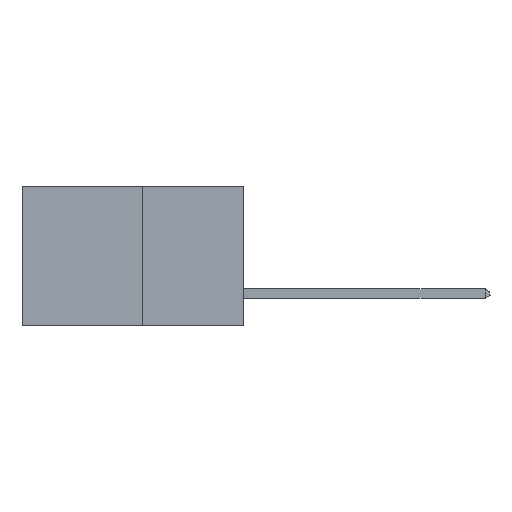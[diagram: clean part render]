
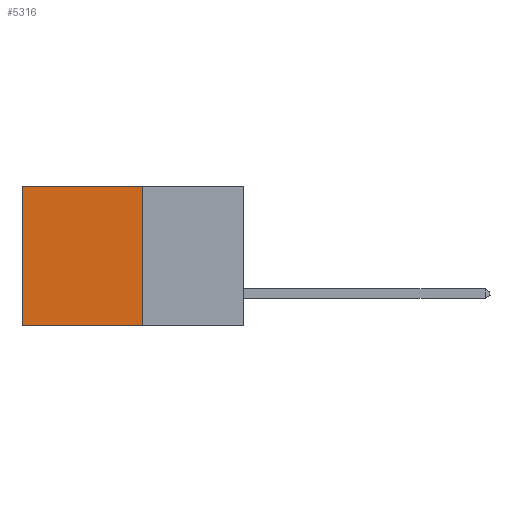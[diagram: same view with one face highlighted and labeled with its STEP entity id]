
A CAD part, left-side view. The second image highlights one B-rep face of the part: STEP entity #5316.
In plain terms, the highlighted planar face has unit normal (-1, 0, 0).
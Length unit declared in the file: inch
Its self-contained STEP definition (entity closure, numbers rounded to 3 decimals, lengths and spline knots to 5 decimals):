
#2037 = DIRECTION ( 'NONE',  ( 0., 0., -1. ) ) ;
#2765 = LINE ( 'NONE', #18623, #16730 ) ;
#3274 = ORIENTED_EDGE ( 'NONE', *, *, #3331, .T. ) ;
#3331 = EDGE_CURVE ( 'NONE', #10796, #9456, #19341, .T. ) ;
#3880 = EDGE_CURVE ( 'NONE', #13641, #21394, #17955, .T. ) ;
#4308 = FACE_OUTER_BOUND ( 'NONE', #7046, .T. ) ;
#5316 = ADVANCED_FACE ( 'NONE', ( #4308 ), #15536, .F. ) ;
#5836 = CARTESIAN_POINT ( 'NONE',  ( 0.277, 0.59, -0.37 ) ) ;
#7046 = EDGE_LOOP ( 'NONE', ( #3274, #19490, #17551, #21540 ) ) ;
#7823 = DIRECTION ( 'NONE',  ( 0., 1., 0. ) ) ;
#9456 = VERTEX_POINT ( 'NONE', #14507 ) ;
#9667 = VECTOR ( 'NONE', #21950, 39.37008 ) ;
#10212 = CARTESIAN_POINT ( 'NONE',  ( 0.277, 0.27, 0. ) ) ;
#10796 = VERTEX_POINT ( 'NONE', #14451 ) ;
#11506 = DIRECTION ( 'NONE',  ( 0., 0., -1. ) ) ;
#11663 = DIRECTION ( 'NONE',  ( 1., 0., 0. ) ) ;
#12351 = CARTESIAN_POINT ( 'NONE',  ( 0.277, 0.27, -0.37 ) ) ;
#13641 = VERTEX_POINT ( 'NONE', #10212 ) ;
#14451 = CARTESIAN_POINT ( 'NONE',  ( 0.277, 0.59, 0. ) ) ;
#14507 = CARTESIAN_POINT ( 'NONE',  ( 0.277, 0.59, -0.37 ) ) ;
#15536 = PLANE ( 'NONE',  #17037 ) ;
#15633 = DIRECTION ( 'NONE',  ( 0., 0., -1. ) ) ;
#16730 = VECTOR ( 'NONE', #7823, 39.37008 ) ;
#17037 = AXIS2_PLACEMENT_3D ( 'NONE', #12351, #11663, #11506 ) ;
#17390 = VECTOR ( 'NONE', #2037, 39.37008 ) ;
#17551 = ORIENTED_EDGE ( 'NONE', *, *, #3880, .F. ) ;
#17955 = LINE ( 'NONE', #20009, #17390 ) ;
#18020 = CARTESIAN_POINT ( 'NONE',  ( 0.277, 0.27, -0.37 ) ) ;
#18623 = CARTESIAN_POINT ( 'NONE',  ( 0.277, 0.27, -0.37 ) ) ;
#18783 = VECTOR ( 'NONE', #15633, 39.37008 ) ;
#19043 = EDGE_CURVE ( 'NONE', #21394, #9456, #2765, .T. ) ;
#19226 = LINE ( 'NONE', #20123, #9667 ) ;
#19341 = LINE ( 'NONE', #5836, #18783 ) ;
#19490 = ORIENTED_EDGE ( 'NONE', *, *, #19043, .F. ) ;
#19563 = EDGE_CURVE ( 'NONE', #13641, #10796, #19226, .T. ) ;
#20009 = CARTESIAN_POINT ( 'NONE',  ( 0.277, 0.27, -0.37 ) ) ;
#20123 = CARTESIAN_POINT ( 'NONE',  ( 0.277, 0.27, 0. ) ) ;
#21394 = VERTEX_POINT ( 'NONE', #18020 ) ;
#21540 = ORIENTED_EDGE ( 'NONE', *, *, #19563, .T. ) ;
#21950 = DIRECTION ( 'NONE',  ( 0., 1., 0. ) ) ;
